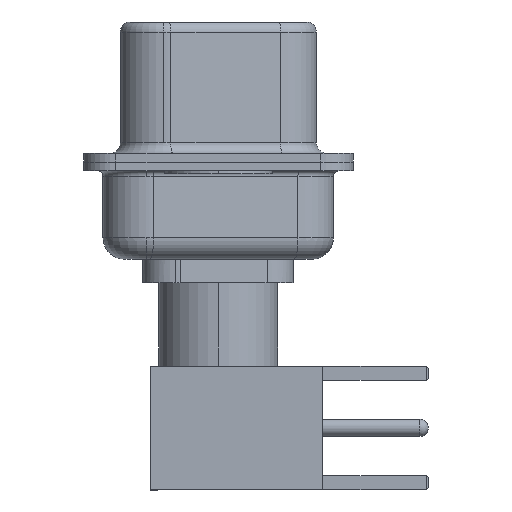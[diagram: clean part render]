
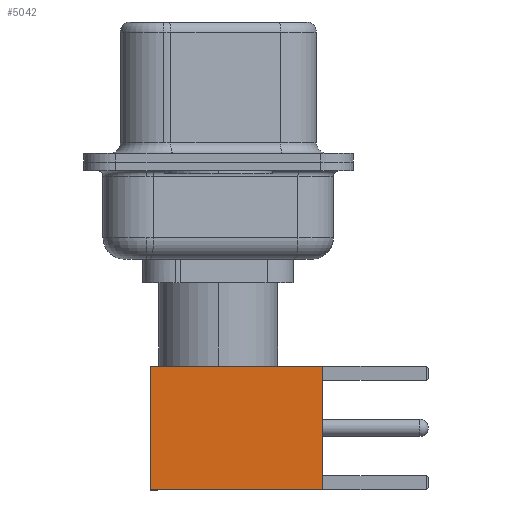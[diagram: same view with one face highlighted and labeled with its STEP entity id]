
A CAD part, left-side view. The second image highlights one B-rep face of the part: STEP entity #5042.
In plain terms, the highlighted face is planar.
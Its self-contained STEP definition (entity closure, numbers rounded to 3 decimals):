
#1010 = DIRECTION ( 'NONE',  ( 0., 0., -1. ) ) ;
#1067 = CARTESIAN_POINT ( 'NONE',  ( -2.875, 2.875, 0. ) ) ;
#1367 = CARTESIAN_POINT ( 'NONE',  ( 0., 2.875, 0. ) ) ;
#1454 = DIRECTION ( 'NONE',  ( 0., 0., -1. ) ) ;
#2554 = CARTESIAN_POINT ( 'NONE',  ( 2.875, 2.875, 0. ) ) ;
#2622 = VECTOR ( 'NONE', #1010, 1000. ) ;
#2731 = DIRECTION ( 'NONE',  ( 0., 0., 1. ) ) ;
#3775 = LINE ( 'NONE', #12003, #2622 ) ;
#3990 = DIRECTION ( 'NONE',  ( 0., 1., 0. ) ) ;
#4084 = CARTESIAN_POINT ( 'NONE',  ( -2.875, 2.875, 8. ) ) ;
#5042 = ADVANCED_FACE ( 'NONE', ( #14827 ), #16363, .T. ) ;
#5547 = ORIENTED_EDGE ( 'NONE', *, *, #6011, .F. ) ;
#6011 = EDGE_CURVE ( 'NONE', #14206, #14601, #6570, .T. ) ;
#6507 = EDGE_LOOP ( 'NONE', ( #16928, #10382, #7113, #5547 ) ) ;
#6570 = LINE ( 'NONE', #14615, #15998 ) ;
#6763 = DIRECTION ( 'NONE',  ( -1., 0., 0. ) ) ;
#7113 = ORIENTED_EDGE ( 'NONE', *, *, #15776, .F. ) ;
#7844 = DIRECTION ( 'NONE',  ( -1., 0., 0. ) ) ;
#9470 = LINE ( 'NONE', #10747, #15579 ) ;
#9489 = CARTESIAN_POINT ( 'NONE',  ( 2.875, 2.875, 0. ) ) ;
#10382 = ORIENTED_EDGE ( 'NONE', *, *, #15826, .T. ) ;
#10747 = CARTESIAN_POINT ( 'NONE',  ( 2.875, 2.875, 0. ) ) ;
#10831 = AXIS2_PLACEMENT_3D ( 'NONE', #2554, #3990, #2731 ) ;
#11622 = EDGE_CURVE ( 'NONE', #14206, #17346, #9470, .T. ) ;
#12003 = CARTESIAN_POINT ( 'NONE',  ( -2.875, 2.875, 0. ) ) ;
#12537 = VERTEX_POINT ( 'NONE', #1067 ) ;
#14206 = VERTEX_POINT ( 'NONE', #15575 ) ;
#14601 = VERTEX_POINT ( 'NONE', #4084 ) ;
#14615 = CARTESIAN_POINT ( 'NONE',  ( 0., 2.875, 8. ) ) ;
#14827 = FACE_OUTER_BOUND ( 'NONE', #6507, .T. ) ;
#15575 = CARTESIAN_POINT ( 'NONE',  ( 2.875, 2.875, 8. ) ) ;
#15579 = VECTOR ( 'NONE', #1454, 1000. ) ;
#15776 = EDGE_CURVE ( 'NONE', #14601, #12537, #3775, .T. ) ;
#15826 = EDGE_CURVE ( 'NONE', #17346, #12537, #17775, .T. ) ;
#15998 = VECTOR ( 'NONE', #7844, 1000. ) ;
#16363 = PLANE ( 'NONE',  #10831 ) ;
#16928 = ORIENTED_EDGE ( 'NONE', *, *, #11622, .T. ) ;
#17328 = VECTOR ( 'NONE', #6763, 1000. ) ;
#17346 = VERTEX_POINT ( 'NONE', #9489 ) ;
#17775 = LINE ( 'NONE', #1367, #17328 ) ;
